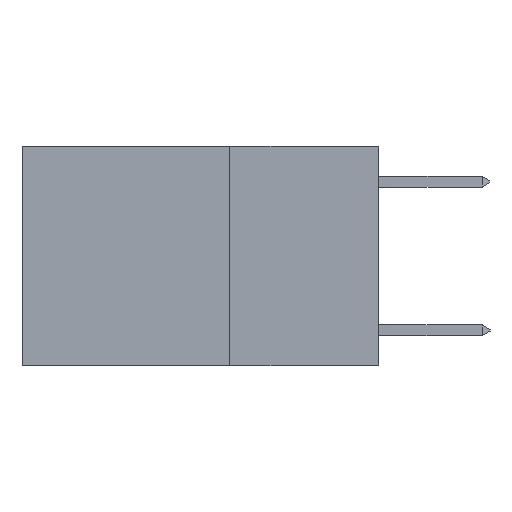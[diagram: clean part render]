
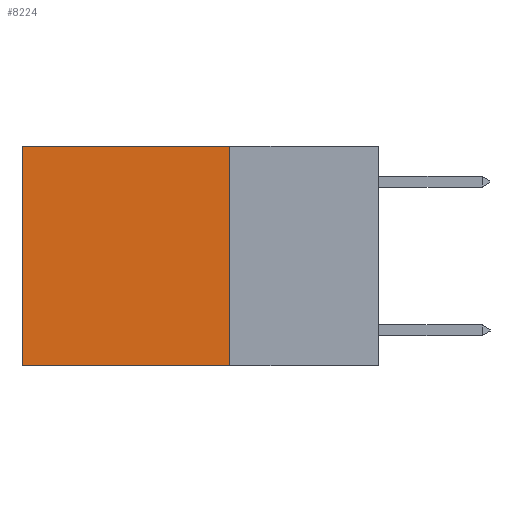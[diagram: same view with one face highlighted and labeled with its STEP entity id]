
A CAD part, left-side view. The second image highlights one B-rep face of the part: STEP entity #8224.
In plain terms, the highlighted planar face has unit normal (-1, 0, 0).
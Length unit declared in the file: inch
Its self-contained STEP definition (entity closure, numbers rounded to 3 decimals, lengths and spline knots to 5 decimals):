
#213 = ORIENTED_EDGE ( 'NONE', *, *, #3402, .T. ) ;
#263 = CARTESIAN_POINT ( 'NONE',  ( 0.2625, 0.6, 0. ) ) ;
#315 = CARTESIAN_POINT ( 'NONE',  ( 0.2625, 0.25, 0. ) ) ;
#713 = CARTESIAN_POINT ( 'NONE',  ( 0.2625, 0.25, 0. ) ) ;
#749 = ORIENTED_EDGE ( 'NONE', *, *, #6903, .F. ) ;
#945 = VERTEX_POINT ( 'NONE', #263 ) ;
#1021 = CARTESIAN_POINT ( 'NONE',  ( 0.2625, 0.6, 0. ) ) ;
#1478 = LINE ( 'NONE', #4690, #3249 ) ;
#1493 = DIRECTION ( 'NONE',  ( 0., 0., -1. ) ) ;
#1824 = VECTOR ( 'NONE', #3310, 39.37008 ) ;
#2541 = CARTESIAN_POINT ( 'NONE',  ( 0.2625, 0.25, 0. ) ) ;
#2608 = DIRECTION ( 'NONE',  ( 0., 0., -1. ) ) ;
#3249 = VECTOR ( 'NONE', #6256, 39.37008 ) ;
#3310 = DIRECTION ( 'NONE',  ( 0., 0., -1. ) ) ;
#3402 = EDGE_CURVE ( 'NONE', #945, #3437, #4343, .T. ) ;
#3437 = VERTEX_POINT ( 'NONE', #7995 ) ;
#3909 = EDGE_CURVE ( 'NONE', #6018, #6280, #5181, .T. ) ;
#3958 = EDGE_LOOP ( 'NONE', ( #213, #749, #4632, #8223 ) ) ;
#4343 = LINE ( 'NONE', #1021, #1824 ) ;
#4632 = ORIENTED_EDGE ( 'NONE', *, *, #3909, .F. ) ;
#4690 = CARTESIAN_POINT ( 'NONE',  ( 0.2625, 0.25, 0. ) ) ;
#4942 = VECTOR ( 'NONE', #1493, 39.37008 ) ;
#5181 = LINE ( 'NONE', #713, #4942 ) ;
#5678 = CARTESIAN_POINT ( 'NONE',  ( 0.2625, 0.25, -0.37 ) ) ;
#6018 = VERTEX_POINT ( 'NONE', #2541 ) ;
#6256 = DIRECTION ( 'NONE',  ( 0., 1., 0. ) ) ;
#6280 = VERTEX_POINT ( 'NONE', #7545 ) ;
#6451 = DIRECTION ( 'NONE',  ( 0., 1., 0. ) ) ;
#6903 = EDGE_CURVE ( 'NONE', #6280, #3437, #7286, .T. ) ;
#7144 = AXIS2_PLACEMENT_3D ( 'NONE', #315, #7240, #2608 ) ;
#7240 = DIRECTION ( 'NONE',  ( 1., 0., 0. ) ) ;
#7286 = LINE ( 'NONE', #5678, #9533 ) ;
#7545 = CARTESIAN_POINT ( 'NONE',  ( 0.2625, 0.25, -0.37 ) ) ;
#7995 = CARTESIAN_POINT ( 'NONE',  ( 0.2625, 0.6, -0.37 ) ) ;
#8036 = EDGE_CURVE ( 'NONE', #6018, #945, #1478, .T. ) ;
#8223 = ORIENTED_EDGE ( 'NONE', *, *, #8036, .T. ) ;
#8224 = ADVANCED_FACE ( 'NONE', ( #9503 ), #9491, .F. ) ;
#9491 = PLANE ( 'NONE',  #7144 ) ;
#9503 = FACE_OUTER_BOUND ( 'NONE', #3958, .T. ) ;
#9533 = VECTOR ( 'NONE', #6451, 39.37008 ) ;
